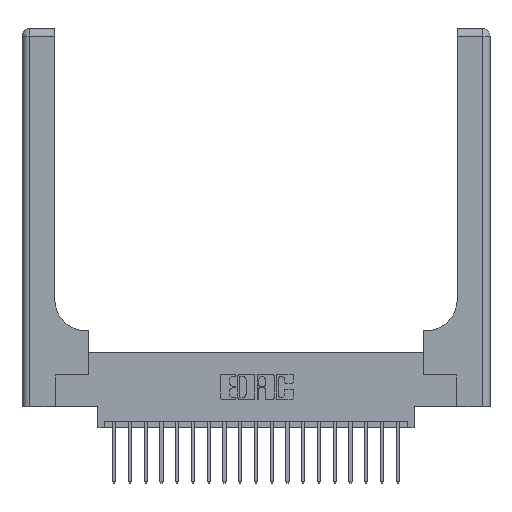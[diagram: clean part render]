
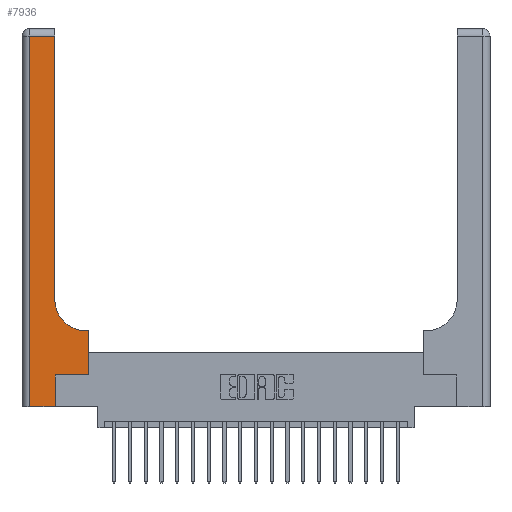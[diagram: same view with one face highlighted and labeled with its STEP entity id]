
A CAD part, top view. The second image highlights one B-rep face of the part: STEP entity #7936.
In plain terms, the highlighted planar face has unit normal (0, 0, 1).
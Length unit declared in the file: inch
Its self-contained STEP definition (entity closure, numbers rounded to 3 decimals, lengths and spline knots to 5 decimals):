
#23 = LINE ( 'NONE', #19836, #9695 ) ;
#157 = LINE ( 'NONE', #9935, #8708 ) ;
#169 = EDGE_CURVE ( 'NONE', #18071, #14736, #21258, .T. ) ;
#566 = VERTEX_POINT ( 'NONE', #1233 ) ;
#748 = DIRECTION ( 'NONE',  ( 0., 0., -1. ) ) ;
#973 = EDGE_CURVE ( 'NONE', #20352, #566, #17902, .T. ) ;
#982 = CARTESIAN_POINT ( 'NONE',  ( 0.06, 2.94, 0.37 ) ) ;
#1233 = CARTESIAN_POINT ( 'NONE',  ( 0.26, 0.85, 0.37 ) ) ;
#1361 = EDGE_CURVE ( 'NONE', #14736, #9744, #20751, .T. ) ;
#2609 = ORIENTED_EDGE ( 'NONE', *, *, #3211, .T. ) ;
#3129 = EDGE_CURVE ( 'NONE', #15837, #11072, #7981, .T. ) ;
#3211 = EDGE_CURVE ( 'NONE', #566, #12414, #23, .T. ) ;
#3947 = EDGE_CURVE ( 'NONE', #11072, #8591, #157, .T. ) ;
#3966 = FACE_OUTER_BOUND ( 'NONE', #9769, .T. ) ;
#4484 = CARTESIAN_POINT ( 'NONE',  ( 0.265, 0., 0.37 ) ) ;
#4893 = DIRECTION ( 'NONE',  ( 1., 0., 0. ) ) ;
#5495 = VECTOR ( 'NONE', #5781, 39.37008 ) ;
#5547 = DIRECTION ( 'NONE',  ( -1., 0., 0. ) ) ;
#5781 = DIRECTION ( 'NONE',  ( 1., 0., 0. ) ) ;
#6896 = EDGE_CURVE ( 'NONE', #12414, #18071, #16957, .T. ) ;
#7142 = LINE ( 'NONE', #20418, #7250 ) ;
#7250 = VECTOR ( 'NONE', #5547, 39.37008 ) ;
#7842 = CARTESIAN_POINT ( 'NONE',  ( 0.265, 0.25, 0.37 ) ) ;
#7936 = ADVANCED_FACE ( 'NONE', ( #3966 ), #18701, .F. ) ;
#7975 = CARTESIAN_POINT ( 'NONE',  ( 0.51, 0.6, 0.37 ) ) ;
#7981 = LINE ( 'NONE', #17921, #14899 ) ;
#8297 = CARTESIAN_POINT ( 'NONE',  ( 0.265, 0., 0.37 ) ) ;
#8591 = VERTEX_POINT ( 'NONE', #18527 ) ;
#8708 = VECTOR ( 'NONE', #10165, 39.37008 ) ;
#8863 = ORIENTED_EDGE ( 'NONE', *, *, #6896, .T. ) ;
#9337 = DIRECTION ( 'NONE',  ( 1., 0., 0. ) ) ;
#9539 = ORIENTED_EDGE ( 'NONE', *, *, #15097, .T. ) ;
#9695 = VECTOR ( 'NONE', #19526, 39.37008 ) ;
#9744 = VERTEX_POINT ( 'NONE', #4484 ) ;
#9769 = EDGE_LOOP ( 'NONE', ( #2609, #8863, #20982, #15099, #16851, #15946, #14166, #9539, #19278 ) ) ;
#9935 = CARTESIAN_POINT ( 'NONE',  ( 0.528, 0.25, 0.37 ) ) ;
#10165 = DIRECTION ( 'NONE',  ( 0., 1., 0. ) ) ;
#10514 = DIRECTION ( 'NONE',  ( 0., 0., -1. ) ) ;
#11072 = VERTEX_POINT ( 'NONE', #18537 ) ;
#11074 = EDGE_CURVE ( 'NONE', #9744, #15837, #16557, .T. ) ;
#12414 = VERTEX_POINT ( 'NONE', #20179 ) ;
#12897 = CARTESIAN_POINT ( 'NONE',  ( 0.06, 3., 0.37 ) ) ;
#13030 = VECTOR ( 'NONE', #17635, 39.37008 ) ;
#13430 = AXIS2_PLACEMENT_3D ( 'NONE', #17563, #748, #9337 ) ;
#14166 = ORIENTED_EDGE ( 'NONE', *, *, #3947, .T. ) ;
#14202 = AXIS2_PLACEMENT_3D ( 'NONE', #19126, #10514, #15600 ) ;
#14736 = VERTEX_POINT ( 'NONE', #16912 ) ;
#14826 = VECTOR ( 'NONE', #15436, 39.37008 ) ;
#14899 = VECTOR ( 'NONE', #4893, 39.37008 ) ;
#14918 = DIRECTION ( 'NONE',  ( 0., 1., 0. ) ) ;
#15085 = VECTOR ( 'NONE', #14918, 39.37008 ) ;
#15097 = EDGE_CURVE ( 'NONE', #8591, #20352, #7142, .T. ) ;
#15099 = ORIENTED_EDGE ( 'NONE', *, *, #1361, .T. ) ;
#15436 = DIRECTION ( 'NONE',  ( -1., 0., 0. ) ) ;
#15600 = DIRECTION ( 'NONE',  ( -1., 0., 0. ) ) ;
#15837 = VERTEX_POINT ( 'NONE', #7842 ) ;
#15946 = ORIENTED_EDGE ( 'NONE', *, *, #3129, .T. ) ;
#16557 = LINE ( 'NONE', #8297, #15085 ) ;
#16851 = ORIENTED_EDGE ( 'NONE', *, *, #11074, .T. ) ;
#16912 = CARTESIAN_POINT ( 'NONE',  ( 0.06, 0., 0.37 ) ) ;
#16957 = LINE ( 'NONE', #18342, #14826 ) ;
#17563 = CARTESIAN_POINT ( 'NONE',  ( 0.51, 0.85, 0.37 ) ) ;
#17635 = DIRECTION ( 'NONE',  ( 0., -1., 0. ) ) ;
#17902 = CIRCLE ( 'NONE', #13430, 0.25 ) ;
#17921 = CARTESIAN_POINT ( 'NONE',  ( 0.265, 0.25, 0.37 ) ) ;
#18071 = VERTEX_POINT ( 'NONE', #982 ) ;
#18342 = CARTESIAN_POINT ( 'NONE',  ( 0., 2.94, 0.37 ) ) ;
#18527 = CARTESIAN_POINT ( 'NONE',  ( 0.528, 0.6, 0.37 ) ) ;
#18537 = CARTESIAN_POINT ( 'NONE',  ( 0.528, 0.25, 0.37 ) ) ;
#18701 = PLANE ( 'NONE',  #14202 ) ;
#19126 = CARTESIAN_POINT ( 'NONE',  ( 0., 3., 0.37 ) ) ;
#19278 = ORIENTED_EDGE ( 'NONE', *, *, #973, .T. ) ;
#19526 = DIRECTION ( 'NONE',  ( 0., 1., 0. ) ) ;
#19836 = CARTESIAN_POINT ( 'NONE',  ( 0.26, 3., 0.37 ) ) ;
#20179 = CARTESIAN_POINT ( 'NONE',  ( 0.26, 2.94, 0.37 ) ) ;
#20352 = VERTEX_POINT ( 'NONE', #7975 ) ;
#20418 = CARTESIAN_POINT ( 'NONE',  ( 0.26, 0.6, 0.37 ) ) ;
#20538 = CARTESIAN_POINT ( 'NONE',  ( 0., 0., 0.37 ) ) ;
#20751 = LINE ( 'NONE', #20538, #5495 ) ;
#20982 = ORIENTED_EDGE ( 'NONE', *, *, #169, .T. ) ;
#21258 = LINE ( 'NONE', #12897, #13030 ) ;
